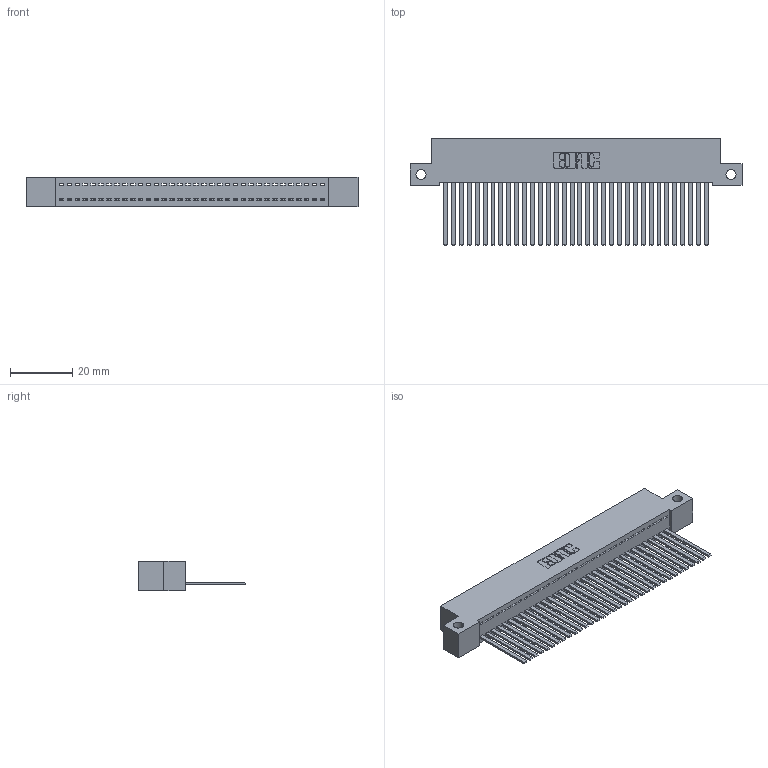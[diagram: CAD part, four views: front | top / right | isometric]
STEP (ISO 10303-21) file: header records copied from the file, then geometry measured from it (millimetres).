
FILE_DESCRIPTION (( 'STEP AP203' ), '1' );
FILE_NAME ('342-034-544-112.STEP', '2019-10-02T12:24:04', ( '' ), ( '' ), 'SwSTEP 2.0', 'SolidWorks 2016', '' );
FILE_SCHEMA (( 'CONFIG_CONTROL_DESIGN' ));
Length unit declared in the file: inch
Products named in the file (3): 342 Part_Side Mount; 345-292-001_345-293-144; 342-034-544-112
Assembly tree (35 placements, depth 2):
  342-034-544-112
    342 Part_Side Mount
    345-292-001_345-293-144  x34
Bounding box: 106.68 x 34.3 x 9.4 mm (x, y, z)
Volume: 9644.1 mm3; surface area: 14970.1 mm2
Topology: 35 solids, 35 shells, 1878 faces, 5671 edges, 3734 vertices
Faces by surface type: plane 1358, cylinder 520
Entity records: 21507 total; most frequent: CARTESIAN_POINT 3716, ORIENTED_EDGE 3686, DIRECTION 3147, EDGE_CURVE 1843, VECTOR 1719, LINE 1719, VERTEX_POINT 1226, AXIS2_PLACEMENT_3D 714
